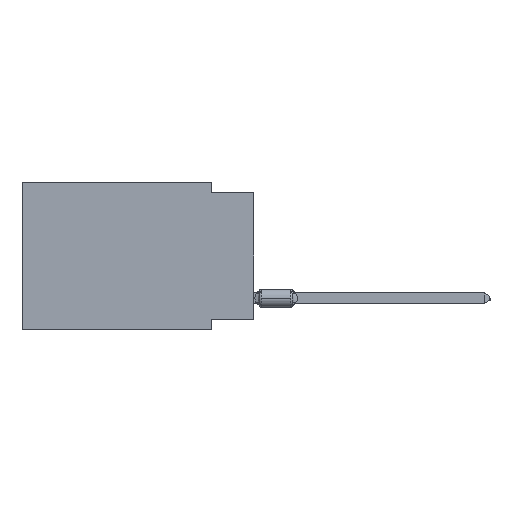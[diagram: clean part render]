
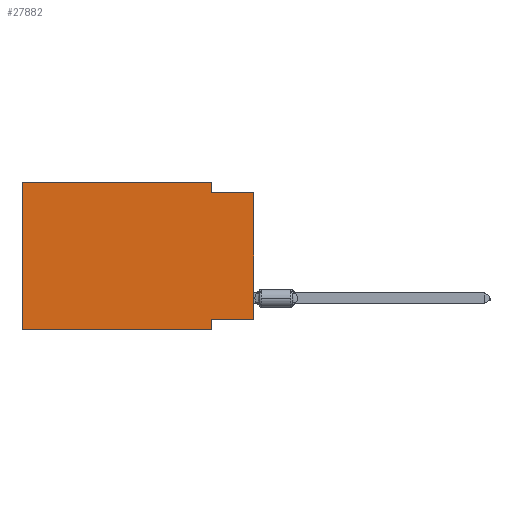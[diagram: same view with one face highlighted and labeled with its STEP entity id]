
A CAD part, left-side view. The second image highlights one B-rep face of the part: STEP entity #27882.
In plain terms, the highlighted planar face has unit normal (-1, 0, 0).
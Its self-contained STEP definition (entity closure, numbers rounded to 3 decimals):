
#450 = ORIENTED_EDGE ( 'NONE', *, *, #16789, .F. ) ;
#762 = DIRECTION ( 'NONE',  ( 0., -1., 0. ) ) ;
#844 = ORIENTED_EDGE ( 'NONE', *, *, #14915, .F. ) ;
#1064 = LINE ( 'NONE', #19979, #13443 ) ;
#1096 = VERTEX_POINT ( 'NONE', #4916 ) ;
#3982 = DIRECTION ( 'NONE',  ( 0., 0., -1. ) ) ;
#3992 = DIRECTION ( 'NONE',  ( 0., 0., -1. ) ) ;
#4916 = CARTESIAN_POINT ( 'NONE',  ( 0., 2.54, -8.255 ) ) ;
#5261 = EDGE_LOOP ( 'NONE', ( #27029, #450, #7714, #12434, #18727, #6283, #844, #26014 ) ) ;
#5855 = VERTEX_POINT ( 'NONE', #16191 ) ;
#6134 = CARTESIAN_POINT ( 'NONE',  ( 0., 13.97, -8.89 ) ) ;
#6283 = ORIENTED_EDGE ( 'NONE', *, *, #8890, .T. ) ;
#6374 = CARTESIAN_POINT ( 'NONE',  ( 0., 13.97, 0. ) ) ;
#6831 = PLANE ( 'NONE',  #10159 ) ;
#7083 = CARTESIAN_POINT ( 'NONE',  ( 0., 2.54, 0. ) ) ;
#7171 = CARTESIAN_POINT ( 'NONE',  ( 0., 13.97, 0. ) ) ;
#7714 = ORIENTED_EDGE ( 'NONE', *, *, #25199, .F. ) ;
#7915 = DIRECTION ( 'NONE',  ( 0., -1., 0. ) ) ;
#8666 = DIRECTION ( 'NONE',  ( 0., 0., -1. ) ) ;
#8890 = EDGE_CURVE ( 'NONE', #15393, #23505, #17159, .T. ) ;
#10138 = CARTESIAN_POINT ( 'NONE',  ( 0., 0., -0.635 ) ) ;
#10159 = AXIS2_PLACEMENT_3D ( 'NONE', #6374, #10986, #8666 ) ;
#10986 = DIRECTION ( 'NONE',  ( 1., 0., 0. ) ) ;
#12405 = EDGE_CURVE ( 'NONE', #15393, #16725, #14997, .T. ) ;
#12434 = ORIENTED_EDGE ( 'NONE', *, *, #29183, .F. ) ;
#12483 = LINE ( 'NONE', #26511, #28151 ) ;
#13443 = VECTOR ( 'NONE', #22294, 1000. ) ;
#13789 = LINE ( 'NONE', #7171, #20070 ) ;
#13798 = EDGE_CURVE ( 'NONE', #18398, #1096, #1064, .T. ) ;
#14195 = CARTESIAN_POINT ( 'NONE',  ( 0., 2.54, -0.635 ) ) ;
#14906 = LINE ( 'NONE', #10138, #30288 ) ;
#14915 = EDGE_CURVE ( 'NONE', #1096, #23505, #21714, .T. ) ;
#14997 = LINE ( 'NONE', #19774, #25208 ) ;
#15393 = VERTEX_POINT ( 'NONE', #6134 ) ;
#16191 = CARTESIAN_POINT ( 'NONE',  ( 0., 0., -0.635 ) ) ;
#16626 = VERTEX_POINT ( 'NONE', #7083 ) ;
#16725 = VERTEX_POINT ( 'NONE', #28931 ) ;
#16789 = EDGE_CURVE ( 'NONE', #23423, #5855, #14906, .T. ) ;
#17159 = LINE ( 'NONE', #19637, #22889 ) ;
#18398 = VERTEX_POINT ( 'NONE', #22213 ) ;
#18449 = CARTESIAN_POINT ( 'NONE',  ( 0., 2.54, 0. ) ) ;
#18727 = ORIENTED_EDGE ( 'NONE', *, *, #12405, .F. ) ;
#19637 = CARTESIAN_POINT ( 'NONE',  ( 0., 13.97, -8.89 ) ) ;
#19727 = DIRECTION ( 'NONE',  ( 0., 0., 1. ) ) ;
#19774 = CARTESIAN_POINT ( 'NONE',  ( 0., 13.97, 0. ) ) ;
#19979 = CARTESIAN_POINT ( 'NONE',  ( 0., 0., -8.255 ) ) ;
#20070 = VECTOR ( 'NONE', #21032, 1000. ) ;
#20142 = LINE ( 'NONE', #18449, #20386 ) ;
#20386 = VECTOR ( 'NONE', #3992, 1000. ) ;
#20681 = FACE_OUTER_BOUND ( 'NONE', #5261, .T. ) ;
#21032 = DIRECTION ( 'NONE',  ( 0., -1., 0. ) ) ;
#21473 = EDGE_CURVE ( 'NONE', #18398, #5855, #12483, .T. ) ;
#21714 = LINE ( 'NONE', #29842, #25273 ) ;
#22213 = CARTESIAN_POINT ( 'NONE',  ( 0., 0., -8.255 ) ) ;
#22294 = DIRECTION ( 'NONE',  ( 0., 1., 0. ) ) ;
#22889 = VECTOR ( 'NONE', #7915, 1000. ) ;
#23423 = VERTEX_POINT ( 'NONE', #14195 ) ;
#23505 = VERTEX_POINT ( 'NONE', #29845 ) ;
#25199 = EDGE_CURVE ( 'NONE', #16626, #23423, #20142, .T. ) ;
#25208 = VECTOR ( 'NONE', #29173, 1000. ) ;
#25273 = VECTOR ( 'NONE', #3982, 1000. ) ;
#26014 = ORIENTED_EDGE ( 'NONE', *, *, #13798, .F. ) ;
#26511 = CARTESIAN_POINT ( 'NONE',  ( 0., 0., 0. ) ) ;
#27029 = ORIENTED_EDGE ( 'NONE', *, *, #21473, .T. ) ;
#27882 = ADVANCED_FACE ( 'NONE', ( #20681 ), #6831, .F. ) ;
#28151 = VECTOR ( 'NONE', #19727, 1000. ) ;
#28931 = CARTESIAN_POINT ( 'NONE',  ( 0., 13.97, 0. ) ) ;
#29173 = DIRECTION ( 'NONE',  ( 0., 0., 1. ) ) ;
#29183 = EDGE_CURVE ( 'NONE', #16725, #16626, #13789, .T. ) ;
#29842 = CARTESIAN_POINT ( 'NONE',  ( 0., 2.54, -8.89 ) ) ;
#29845 = CARTESIAN_POINT ( 'NONE',  ( 0., 2.54, -8.89 ) ) ;
#30288 = VECTOR ( 'NONE', #762, 1000. ) ;
